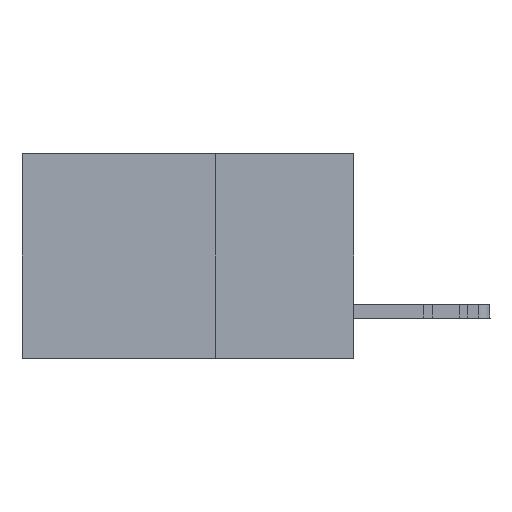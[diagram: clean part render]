
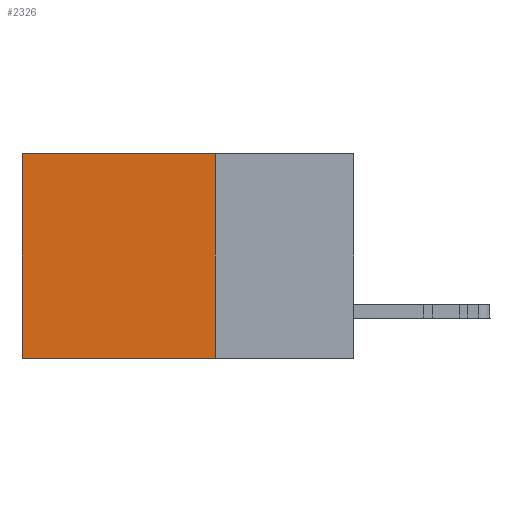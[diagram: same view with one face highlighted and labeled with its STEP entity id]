
A CAD part, left-side view. The second image highlights one B-rep face of the part: STEP entity #2326.
In plain terms, the highlighted planar face has unit normal (-1, 0, 0).
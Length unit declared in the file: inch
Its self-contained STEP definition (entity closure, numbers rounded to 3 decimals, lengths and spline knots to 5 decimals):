
#96 = VECTOR ( 'NONE', #14521, 39.37008 ) ;
#1441 = CARTESIAN_POINT ( 'NONE',  ( 0.2875, 0.25, -0.37 ) ) ;
#1792 = CARTESIAN_POINT ( 'NONE',  ( 0.2875, 0.25, -0.37 ) ) ;
#1902 = ORIENTED_EDGE ( 'NONE', *, *, #2855, .T. ) ;
#2326 = ADVANCED_FACE ( 'NONE', ( #22321 ), #6968, .F. ) ;
#2855 = EDGE_CURVE ( 'NONE', #24457, #28148, #27204, .T. ) ;
#3758 = VECTOR ( 'NONE', #26582, 39.37008 ) ;
#3772 = CARTESIAN_POINT ( 'NONE',  ( 0.2875, 0.25, 0. ) ) ;
#4260 = CARTESIAN_POINT ( 'NONE',  ( 0.2875, 0.6, 0. ) ) ;
#4771 = LINE ( 'NONE', #35986, #3758 ) ;
#6968 = PLANE ( 'NONE',  #22654 ) ;
#7932 = EDGE_CURVE ( 'NONE', #40184, #21076, #4771, .T. ) ;
#8078 = DIRECTION ( 'NONE',  ( 0., 0., -1. ) ) ;
#9100 = ORIENTED_EDGE ( 'NONE', *, *, #29016, .T. ) ;
#9242 = CARTESIAN_POINT ( 'NONE',  ( 0.2875, 0.6, 0. ) ) ;
#11011 = DIRECTION ( 'NONE',  ( 1., 0., 0. ) ) ;
#11630 = CARTESIAN_POINT ( 'NONE',  ( 0.2875, 0.25, 0. ) ) ;
#14521 = DIRECTION ( 'NONE',  ( 0., 1., 0. ) ) ;
#16541 = DIRECTION ( 'NONE',  ( 0., 1., 0. ) ) ;
#16772 = ORIENTED_EDGE ( 'NONE', *, *, #24159, .F. ) ;
#20263 = CARTESIAN_POINT ( 'NONE',  ( 0.2875, 0.25, 0. ) ) ;
#21076 = VERTEX_POINT ( 'NONE', #1441 ) ;
#22321 = FACE_OUTER_BOUND ( 'NONE', #31457, .T. ) ;
#22654 = AXIS2_PLACEMENT_3D ( 'NONE', #20263, #11011, #8078 ) ;
#24159 = EDGE_CURVE ( 'NONE', #21076, #28148, #37534, .T. ) ;
#24293 = CARTESIAN_POINT ( 'NONE',  ( 0.2875, 0.6, -0.37 ) ) ;
#24457 = VERTEX_POINT ( 'NONE', #9242 ) ;
#25313 = VECTOR ( 'NONE', #16541, 39.37008 ) ;
#25935 = VECTOR ( 'NONE', #30169, 39.37008 ) ;
#26582 = DIRECTION ( 'NONE',  ( 0., 0., -1. ) ) ;
#27204 = LINE ( 'NONE', #4260, #25935 ) ;
#28148 = VERTEX_POINT ( 'NONE', #24293 ) ;
#29016 = EDGE_CURVE ( 'NONE', #40184, #24457, #33631, .T. ) ;
#30169 = DIRECTION ( 'NONE',  ( 0., 0., -1. ) ) ;
#30767 = ORIENTED_EDGE ( 'NONE', *, *, #7932, .F. ) ;
#31457 = EDGE_LOOP ( 'NONE', ( #1902, #16772, #30767, #9100 ) ) ;
#33631 = LINE ( 'NONE', #3772, #25313 ) ;
#35986 = CARTESIAN_POINT ( 'NONE',  ( 0.2875, 0.25, 0. ) ) ;
#37534 = LINE ( 'NONE', #1792, #96 ) ;
#40184 = VERTEX_POINT ( 'NONE', #11630 ) ;
